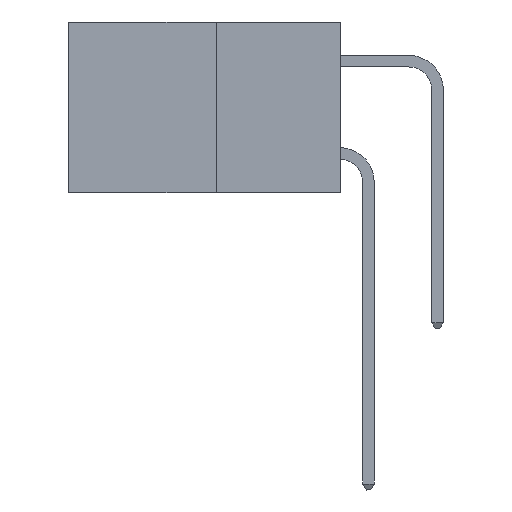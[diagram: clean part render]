
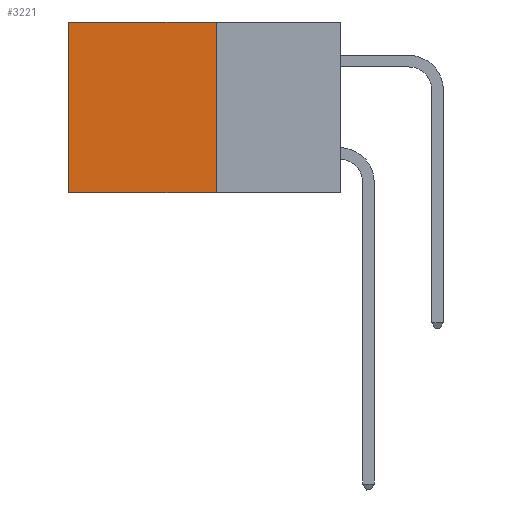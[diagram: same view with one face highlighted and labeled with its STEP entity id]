
A CAD part, left-side view. The second image highlights one B-rep face of the part: STEP entity #3221.
In plain terms, the highlighted planar face has unit normal (-1, 0, 0).
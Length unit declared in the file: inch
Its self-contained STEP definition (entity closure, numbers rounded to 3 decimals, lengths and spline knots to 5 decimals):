
#367 = EDGE_LOOP ( 'NONE', ( #13353, #10594, #1498, #631 ) ) ;
#462 = FACE_OUTER_BOUND ( 'NONE', #367, .T. ) ;
#631 = ORIENTED_EDGE ( 'NONE', *, *, #12982, .T. ) ;
#960 = LINE ( 'NONE', #13370, #8887 ) ;
#1043 = EDGE_CURVE ( 'NONE', #16087, #3146, #3907, .T. ) ;
#1347 = AXIS2_PLACEMENT_3D ( 'NONE', #17786, #4675, #4606 ) ;
#1498 = ORIENTED_EDGE ( 'NONE', *, *, #8204, .F. ) ;
#3094 = DIRECTION ( 'NONE',  ( 0., 1., 0. ) ) ;
#3146 = VERTEX_POINT ( 'NONE', #17890 ) ;
#3221 = ADVANCED_FACE ( 'NONE', ( #462 ), #5403, .F. ) ;
#3907 = LINE ( 'NONE', #5600, #15081 ) ;
#4474 = EDGE_CURVE ( 'NONE', #6270, #3146, #17233, .T. ) ;
#4585 = VERTEX_POINT ( 'NONE', #8601 ) ;
#4606 = DIRECTION ( 'NONE',  ( 0., 0., -1. ) ) ;
#4675 = DIRECTION ( 'NONE',  ( 1., 0., 0. ) ) ;
#5403 = PLANE ( 'NONE',  #1347 ) ;
#5600 = CARTESIAN_POINT ( 'NONE',  ( 0.277, 0.59, -0.37 ) ) ;
#6270 = VERTEX_POINT ( 'NONE', #17427 ) ;
#8204 = EDGE_CURVE ( 'NONE', #4585, #6270, #8773, .T. ) ;
#8601 = CARTESIAN_POINT ( 'NONE',  ( 0.277, 0.27, 0. ) ) ;
#8773 = LINE ( 'NONE', #9217, #15574 ) ;
#8887 = VECTOR ( 'NONE', #3094, 39.37008 ) ;
#9217 = CARTESIAN_POINT ( 'NONE',  ( 0.277, 0.27, -0.37 ) ) ;
#9279 = DIRECTION ( 'NONE',  ( 0., 0., -1. ) ) ;
#10594 = ORIENTED_EDGE ( 'NONE', *, *, #4474, .F. ) ;
#11011 = DIRECTION ( 'NONE',  ( 0., 1., 0. ) ) ;
#11493 = CARTESIAN_POINT ( 'NONE',  ( 0.277, 0.27, -0.37 ) ) ;
#12982 = EDGE_CURVE ( 'NONE', #4585, #16087, #960, .T. ) ;
#13353 = ORIENTED_EDGE ( 'NONE', *, *, #1043, .T. ) ;
#13370 = CARTESIAN_POINT ( 'NONE',  ( 0.277, 0.27, 0. ) ) ;
#13475 = VECTOR ( 'NONE', #11011, 39.37008 ) ;
#15081 = VECTOR ( 'NONE', #18896, 39.37008 ) ;
#15574 = VECTOR ( 'NONE', #9279, 39.37008 ) ;
#15702 = CARTESIAN_POINT ( 'NONE',  ( 0.277, 0.59, 0. ) ) ;
#16087 = VERTEX_POINT ( 'NONE', #15702 ) ;
#17233 = LINE ( 'NONE', #11493, #13475 ) ;
#17427 = CARTESIAN_POINT ( 'NONE',  ( 0.277, 0.27, -0.37 ) ) ;
#17786 = CARTESIAN_POINT ( 'NONE',  ( 0.277, 0.27, -0.37 ) ) ;
#17890 = CARTESIAN_POINT ( 'NONE',  ( 0.277, 0.59, -0.37 ) ) ;
#18896 = DIRECTION ( 'NONE',  ( 0., 0., -1. ) ) ;
